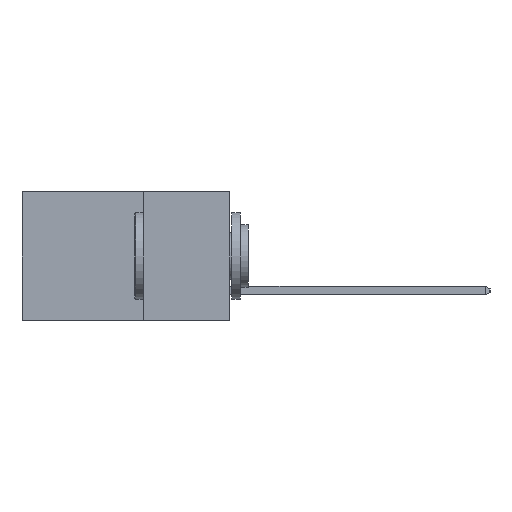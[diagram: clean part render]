
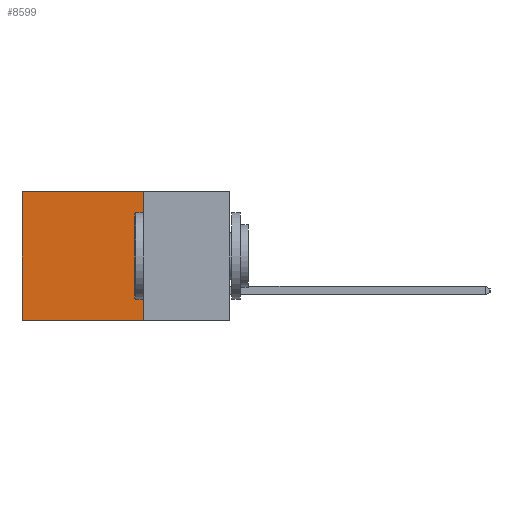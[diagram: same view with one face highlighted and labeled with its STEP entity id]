
A CAD part, left-side view. The second image highlights one B-rep face of the part: STEP entity #8599.
In plain terms, the highlighted planar face has unit normal (-1, 0, 0).
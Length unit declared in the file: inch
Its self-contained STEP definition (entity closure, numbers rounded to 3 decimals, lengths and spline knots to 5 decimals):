
#75 = LINE ( 'NONE', #4761, #373 ) ;
#366 = EDGE_CURVE ( 'NONE', #3972, #863, #3981, .T. ) ;
#373 = VECTOR ( 'NONE', #4749, 39.37008 ) ;
#441 = ORIENTED_EDGE ( 'NONE', *, *, #507, .F. ) ;
#507 = EDGE_CURVE ( 'NONE', #7302, #6164, #6770, .T. ) ;
#863 = VERTEX_POINT ( 'NONE', #1079 ) ;
#1038 = DIRECTION ( 'NONE',  ( 0., 1., 0. ) ) ;
#1079 = CARTESIAN_POINT ( 'NONE',  ( 0.2615, 0.6, 0. ) ) ;
#2358 = DIRECTION ( 'NONE',  ( 0., 0., -1. ) ) ;
#2413 = CARTESIAN_POINT ( 'NONE',  ( 0.2615, 0.25, -0.37 ) ) ;
#3180 = ORIENTED_EDGE ( 'NONE', *, *, #366, .T. ) ;
#3347 = CARTESIAN_POINT ( 'NONE',  ( 0.2615, 0.25, -0.37 ) ) ;
#3764 = CARTESIAN_POINT ( 'NONE',  ( 0.2615, 0.6, -0.37 ) ) ;
#3972 = VERTEX_POINT ( 'NONE', #6658 ) ;
#3973 = DIRECTION ( 'NONE',  ( 0., 0., -1. ) ) ;
#3974 = DIRECTION ( 'NONE',  ( 1., 0., 0. ) ) ;
#3981 = LINE ( 'NONE', #6172, #8006 ) ;
#3989 = CARTESIAN_POINT ( 'NONE',  ( 0.2615, 0.25, -0.37 ) ) ;
#3998 = PLANE ( 'NONE',  #6579 ) ;
#4655 = VECTOR ( 'NONE', #1038, 39.37008 ) ;
#4749 = DIRECTION ( 'NONE',  ( 0., 0., -1. ) ) ;
#4761 = CARTESIAN_POINT ( 'NONE',  ( 0.2615, 0.6, -0.37 ) ) ;
#5815 = EDGE_LOOP ( 'NONE', ( #8630, #441, #9331, #3180 ) ) ;
#5983 = EDGE_CURVE ( 'NONE', #863, #6164, #75, .T. ) ;
#6164 = VERTEX_POINT ( 'NONE', #3764 ) ;
#6172 = CARTESIAN_POINT ( 'NONE',  ( 0.2615, 0.25, 0. ) ) ;
#6579 = AXIS2_PLACEMENT_3D ( 'NONE', #3989, #3974, #3973 ) ;
#6658 = CARTESIAN_POINT ( 'NONE',  ( 0.2615, 0.25, 0. ) ) ;
#6770 = LINE ( 'NONE', #3347, #4655 ) ;
#6816 = VECTOR ( 'NONE', #2358, 39.37008 ) ;
#7302 = VERTEX_POINT ( 'NONE', #10637 ) ;
#7700 = FACE_OUTER_BOUND ( 'NONE', #5815, .T. ) ;
#8006 = VECTOR ( 'NONE', #10296, 39.37008 ) ;
#8599 = ADVANCED_FACE ( 'NONE', ( #7700 ), #3998, .F. ) ;
#8630 = ORIENTED_EDGE ( 'NONE', *, *, #5983, .T. ) ;
#8889 = EDGE_CURVE ( 'NONE', #3972, #7302, #9333, .T. ) ;
#9331 = ORIENTED_EDGE ( 'NONE', *, *, #8889, .F. ) ;
#9333 = LINE ( 'NONE', #2413, #6816 ) ;
#10296 = DIRECTION ( 'NONE',  ( 0., 1., 0. ) ) ;
#10637 = CARTESIAN_POINT ( 'NONE',  ( 0.2615, 0.25, -0.37 ) ) ;
